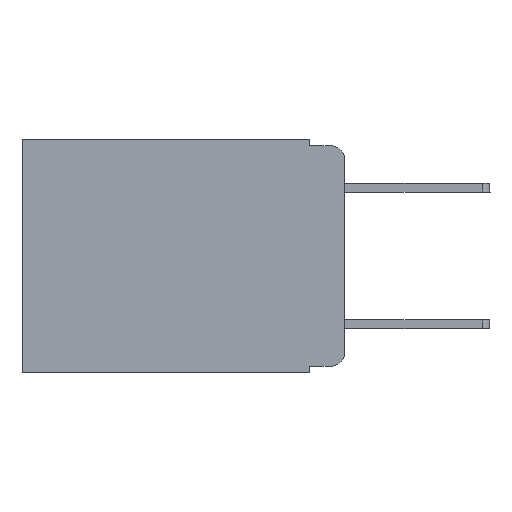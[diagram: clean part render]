
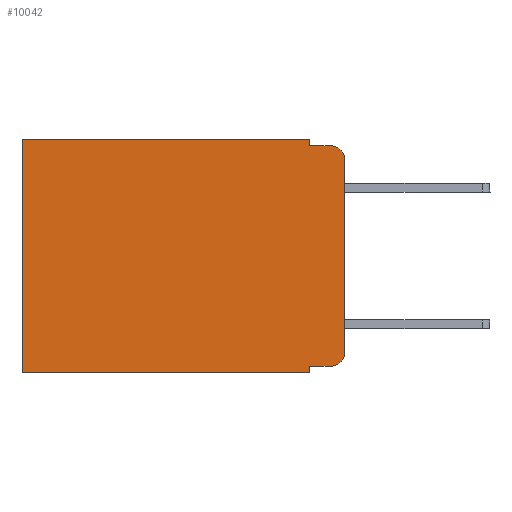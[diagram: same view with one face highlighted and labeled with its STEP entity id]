
A CAD part, left-side view. The second image highlights one B-rep face of the part: STEP entity #10042.
In plain terms, the highlighted planar face has unit normal (-1, 0, 0).
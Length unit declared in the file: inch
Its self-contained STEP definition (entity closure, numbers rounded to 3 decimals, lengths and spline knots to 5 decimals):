
#6 = DIRECTION ( 'NONE',  ( 0., 0., -1. ) ) ;
#46 = EDGE_CURVE ( 'NONE', #8209, #4771, #6263, .T. ) ;
#155 = EDGE_CURVE ( 'NONE', #5102, #5338, #881, .T. ) ;
#196 = AXIS2_PLACEMENT_3D ( 'NONE', #2764, #1082, #4379 ) ;
#344 = LINE ( 'NONE', #1164, #441 ) ;
#402 = LINE ( 'NONE', #4167, #7681 ) ;
#441 = VECTOR ( 'NONE', #9882, 39.37008 ) ;
#548 = VECTOR ( 'NONE', #7883, 39.37008 ) ;
#747 = DIRECTION ( 'NONE',  ( 1., 0., 0. ) ) ;
#881 = LINE ( 'NONE', #2399, #548 ) ;
#1082 = DIRECTION ( 'NONE',  ( -1., 0., 0. ) ) ;
#1164 = CARTESIAN_POINT ( 'NONE',  ( 0.298, 0., -0.343 ) ) ;
#1228 = LINE ( 'NONE', #3585, #9736 ) ;
#2014 = ORIENTED_EDGE ( 'NONE', *, *, #9515, .T. ) ;
#2021 = LINE ( 'NONE', #6869, #4758 ) ;
#2158 = LINE ( 'NONE', #9928, #7181 ) ;
#2304 = DIRECTION ( 'NONE',  ( 0., -1., 0. ) ) ;
#2359 = CIRCLE ( 'NONE', #196, 0.02 ) ;
#2399 = CARTESIAN_POINT ( 'NONE',  ( 0.298, 0.051, -0.01 ) ) ;
#2456 = CIRCLE ( 'NONE', #8239, 0.02 ) ;
#2647 = CARTESIAN_POINT ( 'NONE',  ( 0.298, 0.051, -0.333 ) ) ;
#2674 = CARTESIAN_POINT ( 'NONE',  ( 0.298, 0.051, -0.343 ) ) ;
#2764 = CARTESIAN_POINT ( 'NONE',  ( 0.298, 0.02, -0.03 ) ) ;
#2942 = DIRECTION ( 'NONE',  ( 0., 0., -1. ) ) ;
#2981 = ORIENTED_EDGE ( 'NONE', *, *, #46, .T. ) ;
#3021 = DIRECTION ( 'NONE',  ( -1., 0., 0. ) ) ;
#3099 = EDGE_CURVE ( 'NONE', #4823, #5102, #2021, .T. ) ;
#3109 = VERTEX_POINT ( 'NONE', #8339 ) ;
#3152 = VERTEX_POINT ( 'NONE', #3490 ) ;
#3490 = CARTESIAN_POINT ( 'NONE',  ( 0.298, 0., -0.03 ) ) ;
#3585 = CARTESIAN_POINT ( 'NONE',  ( 0.298, 0.051, 0. ) ) ;
#3587 = DIRECTION ( 'NONE',  ( 0., 1., 0. ) ) ;
#3603 = EDGE_CURVE ( 'NONE', #9047, #8160, #344, .T. ) ;
#3699 = CARTESIAN_POINT ( 'NONE',  ( 0.298, 0.051, 0. ) ) ;
#3788 = CARTESIAN_POINT ( 'NONE',  ( 0.298, 0., 0. ) ) ;
#3843 = PLANE ( 'NONE',  #9178 ) ;
#4167 = CARTESIAN_POINT ( 'NONE',  ( 0.298, 0., 0. ) ) ;
#4204 = VECTOR ( 'NONE', #2304, 39.37008 ) ;
#4379 = DIRECTION ( 'NONE',  ( 0., 0., -1. ) ) ;
#4499 = ORIENTED_EDGE ( 'NONE', *, *, #3099, .F. ) ;
#4518 = DIRECTION ( 'NONE',  ( 0., 0., -1. ) ) ;
#4627 = EDGE_CURVE ( 'NONE', #4771, #3109, #2456, .T. ) ;
#4717 = ORIENTED_EDGE ( 'NONE', *, *, #3603, .F. ) ;
#4758 = VECTOR ( 'NONE', #5937, 39.37008 ) ;
#4771 = VERTEX_POINT ( 'NONE', #5778 ) ;
#4814 = EDGE_CURVE ( 'NONE', #8209, #9047, #1228, .T. ) ;
#4823 = VERTEX_POINT ( 'NONE', #3699 ) ;
#5101 = LINE ( 'NONE', #8227, #8334 ) ;
#5102 = VERTEX_POINT ( 'NONE', #9512 ) ;
#5136 = DIRECTION ( 'NONE',  ( 0., 0., -1. ) ) ;
#5292 = ORIENTED_EDGE ( 'NONE', *, *, #4814, .F. ) ;
#5338 = VERTEX_POINT ( 'NONE', #6178 ) ;
#5778 = CARTESIAN_POINT ( 'NONE',  ( 0.298, 0.02, -0.333 ) ) ;
#5937 = DIRECTION ( 'NONE',  ( 0., 0., -1. ) ) ;
#5942 = VERTEX_POINT ( 'NONE', #6581 ) ;
#6119 = ORIENTED_EDGE ( 'NONE', *, *, #8826, .F. ) ;
#6178 = CARTESIAN_POINT ( 'NONE',  ( 0.298, 0.02, -0.01 ) ) ;
#6263 = LINE ( 'NONE', #9379, #4204 ) ;
#6332 = EDGE_LOOP ( 'NONE', ( #6119, #10174, #8288, #4499, #2014, #10219, #4717, #5292, #2981, #8703 ) ) ;
#6581 = CARTESIAN_POINT ( 'NONE',  ( 0.298, 0.473, 0. ) ) ;
#6869 = CARTESIAN_POINT ( 'NONE',  ( 0.298, 0.051, 0. ) ) ;
#7181 = VECTOR ( 'NONE', #5136, 39.37008 ) ;
#7511 = CARTESIAN_POINT ( 'NONE',  ( 0.298, 0.473, -0.343 ) ) ;
#7644 = FACE_OUTER_BOUND ( 'NONE', #6332, .T. ) ;
#7681 = VECTOR ( 'NONE', #3587, 39.37008 ) ;
#7705 = EDGE_CURVE ( 'NONE', #3152, #5338, #2359, .T. ) ;
#7883 = DIRECTION ( 'NONE',  ( 0., -1., 0. ) ) ;
#8160 = VERTEX_POINT ( 'NONE', #7511 ) ;
#8209 = VERTEX_POINT ( 'NONE', #2647 ) ;
#8227 = CARTESIAN_POINT ( 'NONE',  ( 0.298, 0.473, 0. ) ) ;
#8239 = AXIS2_PLACEMENT_3D ( 'NONE', #10169, #3021, #6 ) ;
#8288 = ORIENTED_EDGE ( 'NONE', *, *, #155, .F. ) ;
#8334 = VECTOR ( 'NONE', #9886, 39.37008 ) ;
#8339 = CARTESIAN_POINT ( 'NONE',  ( 0.298, 0., -0.313 ) ) ;
#8703 = ORIENTED_EDGE ( 'NONE', *, *, #4627, .T. ) ;
#8826 = EDGE_CURVE ( 'NONE', #3152, #3109, #2158, .T. ) ;
#9047 = VERTEX_POINT ( 'NONE', #2674 ) ;
#9178 = AXIS2_PLACEMENT_3D ( 'NONE', #3788, #747, #2942 ) ;
#9379 = CARTESIAN_POINT ( 'NONE',  ( 0.298, 0.051, -0.333 ) ) ;
#9512 = CARTESIAN_POINT ( 'NONE',  ( 0.298, 0.051, -0.01 ) ) ;
#9515 = EDGE_CURVE ( 'NONE', #4823, #5942, #402, .T. ) ;
#9573 = EDGE_CURVE ( 'NONE', #5942, #8160, #5101, .T. ) ;
#9736 = VECTOR ( 'NONE', #4518, 39.37008 ) ;
#9882 = DIRECTION ( 'NONE',  ( 0., 1., 0. ) ) ;
#9886 = DIRECTION ( 'NONE',  ( 0., 0., -1. ) ) ;
#9928 = CARTESIAN_POINT ( 'NONE',  ( 0.298, 0., 0. ) ) ;
#10042 = ADVANCED_FACE ( 'NONE', ( #7644 ), #3843, .F. ) ;
#10169 = CARTESIAN_POINT ( 'NONE',  ( 0.298, 0.02, -0.313 ) ) ;
#10174 = ORIENTED_EDGE ( 'NONE', *, *, #7705, .T. ) ;
#10219 = ORIENTED_EDGE ( 'NONE', *, *, #9573, .T. ) ;
